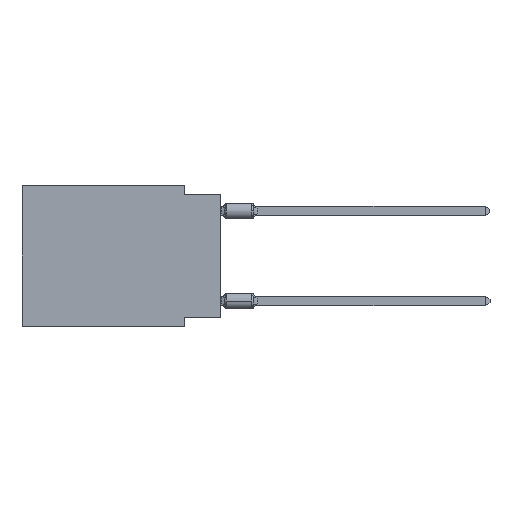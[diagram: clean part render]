
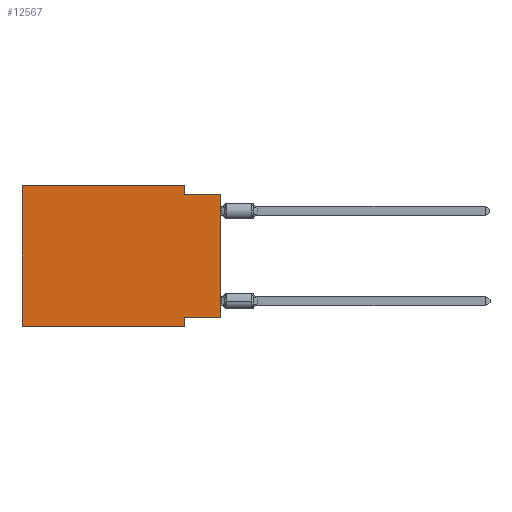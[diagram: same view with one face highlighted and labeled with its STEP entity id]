
A CAD part, left-side view. The second image highlights one B-rep face of the part: STEP entity #12567.
In plain terms, the highlighted planar face has unit normal (-1, 0, 0).
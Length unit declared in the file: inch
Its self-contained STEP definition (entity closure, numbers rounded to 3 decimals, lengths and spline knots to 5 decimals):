
#109 = ORIENTED_EDGE ( 'NONE', *, *, #26075, .F. ) ;
#216 = VERTEX_POINT ( 'NONE', #27412 ) ;
#358 = CARTESIAN_POINT ( 'NONE',  ( 0., 0., -0.025 ) ) ;
#511 = DIRECTION ( 'NONE',  ( 0., 0., -1. ) ) ;
#1760 = EDGE_LOOP ( 'NONE', ( #2498, #23732, #3679, #14514, #24322, #28003, #13633, #109 ) ) ;
#2039 = CARTESIAN_POINT ( 'NONE',  ( 0., 0.55, -0.39 ) ) ;
#2293 = VECTOR ( 'NONE', #6742, 39.37008 ) ;
#2324 = VERTEX_POINT ( 'NONE', #23904 ) ;
#2498 = ORIENTED_EDGE ( 'NONE', *, *, #6414, .T. ) ;
#2669 = LINE ( 'NONE', #4938, #27076 ) ;
#2694 = VECTOR ( 'NONE', #14545, 39.37008 ) ;
#2754 = DIRECTION ( 'NONE',  ( 0., -1., 0. ) ) ;
#3679 = ORIENTED_EDGE ( 'NONE', *, *, #8195, .F. ) ;
#4938 = CARTESIAN_POINT ( 'NONE',  ( 0., 0.1, 0. ) ) ;
#5003 = LINE ( 'NONE', #14195, #23216 ) ;
#5668 = CARTESIAN_POINT ( 'NONE',  ( 0., 0.1, -0.365 ) ) ;
#6320 = VECTOR ( 'NONE', #14449, 39.37008 ) ;
#6414 = EDGE_CURVE ( 'NONE', #10022, #17190, #25611, .T. ) ;
#6742 = DIRECTION ( 'NONE',  ( 0., -1., 0. ) ) ;
#8195 = EDGE_CURVE ( 'NONE', #216, #9969, #2669, .T. ) ;
#8340 = VECTOR ( 'NONE', #13488, 39.37008 ) ;
#8674 = LINE ( 'NONE', #358, #11951 ) ;
#9393 = FACE_OUTER_BOUND ( 'NONE', #1760, .T. ) ;
#9531 = DIRECTION ( 'NONE',  ( 1., 0., 0. ) ) ;
#9823 = PLANE ( 'NONE',  #26801 ) ;
#9969 = VERTEX_POINT ( 'NONE', #12306 ) ;
#9998 = CARTESIAN_POINT ( 'NONE',  ( 0., 0.55, 0. ) ) ;
#10022 = VERTEX_POINT ( 'NONE', #29033 ) ;
#10215 = EDGE_CURVE ( 'NONE', #9969, #17190, #8674, .T. ) ;
#11445 = EDGE_CURVE ( 'NONE', #2324, #216, #11677, .T. ) ;
#11677 = LINE ( 'NONE', #9998, #2694 ) ;
#11951 = VECTOR ( 'NONE', #2754, 39.37008 ) ;
#12306 = CARTESIAN_POINT ( 'NONE',  ( 0., 0.1, -0.025 ) ) ;
#12567 = ADVANCED_FACE ( 'NONE', ( #9393 ), #9823, .F. ) ;
#13250 = EDGE_CURVE ( 'NONE', #22629, #24673, #27519, .T. ) ;
#13488 = DIRECTION ( 'NONE',  ( 0., 0., -1. ) ) ;
#13633 = ORIENTED_EDGE ( 'NONE', *, *, #23802, .F. ) ;
#14195 = CARTESIAN_POINT ( 'NONE',  ( 0., 0., -0.365 ) ) ;
#14449 = DIRECTION ( 'NONE',  ( 0., 0., 1. ) ) ;
#14514 = ORIENTED_EDGE ( 'NONE', *, *, #11445, .F. ) ;
#14545 = DIRECTION ( 'NONE',  ( 0., -1., 0. ) ) ;
#16730 = DIRECTION ( 'NONE',  ( 0., 1., 0. ) ) ;
#17190 = VERTEX_POINT ( 'NONE', #27503 ) ;
#18638 = VERTEX_POINT ( 'NONE', #5668 ) ;
#18662 = CARTESIAN_POINT ( 'NONE',  ( 0., 0., 0. ) ) ;
#19449 = CARTESIAN_POINT ( 'NONE',  ( 0., 0.1, -0.39 ) ) ;
#20468 = LINE ( 'NONE', #25295, #24311 ) ;
#21038 = DIRECTION ( 'NONE',  ( 0., 0., -1. ) ) ;
#22629 = VERTEX_POINT ( 'NONE', #2039 ) ;
#23216 = VECTOR ( 'NONE', #16730, 39.37008 ) ;
#23732 = ORIENTED_EDGE ( 'NONE', *, *, #10215, .F. ) ;
#23802 = EDGE_CURVE ( 'NONE', #18638, #24673, #27500, .T. ) ;
#23904 = CARTESIAN_POINT ( 'NONE',  ( 0., 0.55, 0. ) ) ;
#24311 = VECTOR ( 'NONE', #27263, 39.37008 ) ;
#24322 = ORIENTED_EDGE ( 'NONE', *, *, #29693, .F. ) ;
#24673 = VERTEX_POINT ( 'NONE', #19449 ) ;
#24799 = CARTESIAN_POINT ( 'NONE',  ( 0., 0.55, -0.39 ) ) ;
#25237 = CARTESIAN_POINT ( 'NONE',  ( 0., 0.1, -0.39 ) ) ;
#25295 = CARTESIAN_POINT ( 'NONE',  ( 0., 0.55, 0. ) ) ;
#25611 = LINE ( 'NONE', #18662, #6320 ) ;
#25819 = CARTESIAN_POINT ( 'NONE',  ( 0., 0.55, 0. ) ) ;
#26075 = EDGE_CURVE ( 'NONE', #10022, #18638, #5003, .T. ) ;
#26801 = AXIS2_PLACEMENT_3D ( 'NONE', #25819, #9531, #511 ) ;
#27076 = VECTOR ( 'NONE', #21038, 39.37008 ) ;
#27263 = DIRECTION ( 'NONE',  ( 0., 0., 1. ) ) ;
#27412 = CARTESIAN_POINT ( 'NONE',  ( 0., 0.1, 0. ) ) ;
#27500 = LINE ( 'NONE', #25237, #8340 ) ;
#27503 = CARTESIAN_POINT ( 'NONE',  ( 0., 0., -0.025 ) ) ;
#27519 = LINE ( 'NONE', #24799, #2293 ) ;
#28003 = ORIENTED_EDGE ( 'NONE', *, *, #13250, .T. ) ;
#29033 = CARTESIAN_POINT ( 'NONE',  ( 0., 0., -0.365 ) ) ;
#29693 = EDGE_CURVE ( 'NONE', #22629, #2324, #20468, .T. ) ;
